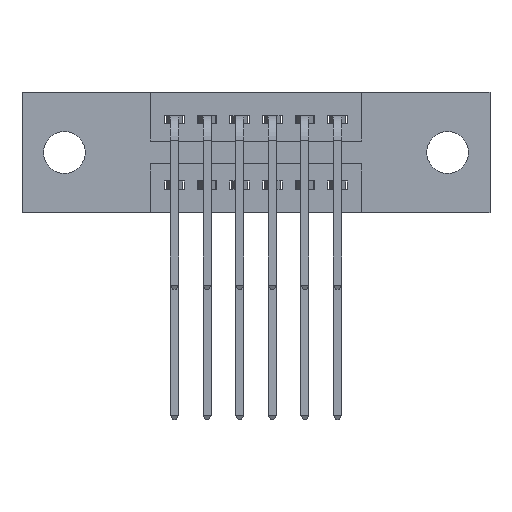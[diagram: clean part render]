
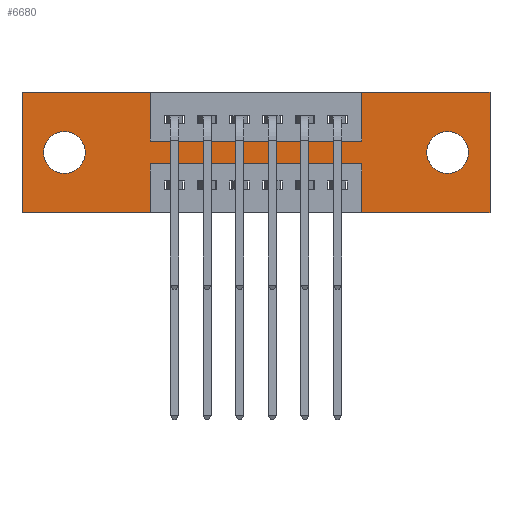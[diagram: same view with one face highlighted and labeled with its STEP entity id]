
A CAD part, front view. The second image highlights one B-rep face of the part: STEP entity #6680.
In plain terms, the highlighted planar face has unit normal (0, -1, 0).
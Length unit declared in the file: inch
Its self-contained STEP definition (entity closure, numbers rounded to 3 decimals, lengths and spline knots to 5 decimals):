
#110 = VERTEX_POINT ( 'NONE', #5980 ) ;
#482 = CARTESIAN_POINT ( 'NONE',  ( 0.13, 0., -0.249 ) ) ;
#796 = DIRECTION ( 'NONE',  ( 0., 0., 1. ) ) ;
#899 = EDGE_LOOP ( 'NONE', ( #6885, #7157 ) ) ;
#951 = DIRECTION ( 'NONE',  ( 0., 1., 0. ) ) ;
#990 = ORIENTED_EDGE ( 'NONE', *, *, #6257, .F. ) ;
#1080 = CARTESIAN_POINT ( 'NONE',  ( 1.305, 0., -0.185 ) ) ;
#1132 = VERTEX_POINT ( 'NONE', #8359 ) ;
#1253 = DIRECTION ( 'NONE',  ( 0., 0., -1. ) ) ;
#1435 = EDGE_LOOP ( 'NONE', ( #5346, #6732 ) ) ;
#1572 = AXIS2_PLACEMENT_3D ( 'NONE', #5475, #6610, #10519 ) ;
#1613 = VERTEX_POINT ( 'NONE', #11039 ) ;
#1637 = CARTESIAN_POINT ( 'NONE',  ( 0.3925, 0., -0.37 ) ) ;
#1645 = LINE ( 'NONE', #7746, #5873 ) ;
#1800 = VECTOR ( 'NONE', #2091, 39.37008 ) ;
#1890 = DIRECTION ( 'NONE',  ( 0., 0., 1. ) ) ;
#1992 = VECTOR ( 'NONE', #7218, 39.37008 ) ;
#2032 = VECTOR ( 'NONE', #8519, 39.37008 ) ;
#2034 = ORIENTED_EDGE ( 'NONE', *, *, #11187, .F. ) ;
#2044 = EDGE_CURVE ( 'NONE', #8488, #10544, #10368, .T. ) ;
#2058 = DIRECTION ( 'NONE',  ( 0., 0., -1. ) ) ;
#2091 = DIRECTION ( 'NONE',  ( 1., 0., 0. ) ) ;
#2223 = CARTESIAN_POINT ( 'NONE',  ( 1.435, 0., 0. ) ) ;
#2295 = VECTOR ( 'NONE', #4329, 39.37008 ) ;
#2473 = DIRECTION ( 'NONE',  ( 0., 0., -1. ) ) ;
#2516 = CARTESIAN_POINT ( 'NONE',  ( 0.13, 0., -0.121 ) ) ;
#2913 = PLANE ( 'NONE',  #1572 ) ;
#2925 = FACE_OUTER_BOUND ( 'NONE', #10430, .T. ) ;
#2967 = CIRCLE ( 'NONE', #6781, 0.064 ) ;
#2994 = VERTEX_POINT ( 'NONE', #9888 ) ;
#3142 = DIRECTION ( 'NONE',  ( 0., 0., 1. ) ) ;
#3173 = VECTOR ( 'NONE', #1890, 39.37008 ) ;
#3327 = CARTESIAN_POINT ( 'NONE',  ( 1.305, 0., -0.185 ) ) ;
#3368 = DIRECTION ( 'NONE',  ( 0., 1., 0. ) ) ;
#3375 = LINE ( 'NONE', #4186, #7590 ) ;
#3460 = LINE ( 'NONE', #7805, #3173 ) ;
#3472 = CARTESIAN_POINT ( 'NONE',  ( 0., 0., -0.37 ) ) ;
#3793 = ORIENTED_EDGE ( 'NONE', *, *, #10353, .F. ) ;
#3949 = AXIS2_PLACEMENT_3D ( 'NONE', #3327, #3368, #2473 ) ;
#4036 = VECTOR ( 'NONE', #6862, 39.37008 ) ;
#4050 = CARTESIAN_POINT ( 'NONE',  ( 0.13, 0., -0.185 ) ) ;
#4064 = CARTESIAN_POINT ( 'NONE',  ( 1.0425, 0., -0.37 ) ) ;
#4069 = ORIENTED_EDGE ( 'NONE', *, *, #7620, .F. ) ;
#4095 = LINE ( 'NONE', #4652, #1800 ) ;
#4186 = CARTESIAN_POINT ( 'NONE',  ( 0.3925, 0., -0.37 ) ) ;
#4329 = DIRECTION ( 'NONE',  ( -1., 0., 0. ) ) ;
#4341 = CARTESIAN_POINT ( 'NONE',  ( 0.3925, 0., -0.22 ) ) ;
#4430 = ORIENTED_EDGE ( 'NONE', *, *, #9631, .F. ) ;
#4598 = EDGE_CURVE ( 'NONE', #8013, #10363, #8521, .T. ) ;
#4652 = CARTESIAN_POINT ( 'NONE',  ( 0.3925, 0., -0.15 ) ) ;
#4670 = CIRCLE ( 'NONE', #8325, 0.064 ) ;
#4731 = CARTESIAN_POINT ( 'NONE',  ( 1.435, 0., 0. ) ) ;
#4863 = VECTOR ( 'NONE', #6016, 39.37008 ) ;
#4864 = DIRECTION ( 'NONE',  ( 0., 0., 1. ) ) ;
#4974 = VERTEX_POINT ( 'NONE', #9897 ) ;
#5029 = VERTEX_POINT ( 'NONE', #2516 ) ;
#5172 = ORIENTED_EDGE ( 'NONE', *, *, #10574, .F. ) ;
#5346 = ORIENTED_EDGE ( 'NONE', *, *, #10771, .T. ) ;
#5475 = CARTESIAN_POINT ( 'NONE',  ( 0., 0., -0.37 ) ) ;
#5684 = ORIENTED_EDGE ( 'NONE', *, *, #7367, .F. ) ;
#5700 = VECTOR ( 'NONE', #3142, 39.37008 ) ;
#5838 = DIRECTION ( 'NONE',  ( 0., 0., -1. ) ) ;
#5873 = VECTOR ( 'NONE', #796, 39.37008 ) ;
#5918 = CARTESIAN_POINT ( 'NONE',  ( 0.3925, 0., -0.22 ) ) ;
#5980 = CARTESIAN_POINT ( 'NONE',  ( 1.435, 0., -0.37 ) ) ;
#6016 = DIRECTION ( 'NONE',  ( 0., 0., -1. ) ) ;
#6097 = CARTESIAN_POINT ( 'NONE',  ( 0.13, 0., -0.185 ) ) ;
#6151 = VERTEX_POINT ( 'NONE', #4341 ) ;
#6163 = LINE ( 'NONE', #6328, #1992 ) ;
#6257 = EDGE_CURVE ( 'NONE', #1613, #7029, #6163, .T. ) ;
#6328 = CARTESIAN_POINT ( 'NONE',  ( 0., 0., 0. ) ) ;
#6338 = CIRCLE ( 'NONE', #10273, 0.064 ) ;
#6579 = CARTESIAN_POINT ( 'NONE',  ( 1.305, 0., -0.249 ) ) ;
#6610 = DIRECTION ( 'NONE',  ( 0., -1., 0. ) ) ;
#6680 = ADVANCED_FACE ( 'NONE', ( #7410, #9677, #2925 ), #2913, .T. ) ;
#6732 = ORIENTED_EDGE ( 'NONE', *, *, #2044, .T. ) ;
#6761 = ORIENTED_EDGE ( 'NONE', *, *, #10606, .F. ) ;
#6781 = AXIS2_PLACEMENT_3D ( 'NONE', #6097, #951, #6973 ) ;
#6862 = DIRECTION ( 'NONE',  ( 1., 0., 0. ) ) ;
#6885 = ORIENTED_EDGE ( 'NONE', *, *, #10942, .T. ) ;
#6973 = DIRECTION ( 'NONE',  ( 0., 0., 1. ) ) ;
#6996 = LINE ( 'NONE', #5918, #2295 ) ;
#7029 = VERTEX_POINT ( 'NONE', #2223 ) ;
#7072 = CARTESIAN_POINT ( 'NONE',  ( 0., 0., 0. ) ) ;
#7079 = DIRECTION ( 'NONE',  ( 0., 1., 0. ) ) ;
#7157 = ORIENTED_EDGE ( 'NONE', *, *, #10693, .T. ) ;
#7218 = DIRECTION ( 'NONE',  ( 1., 0., 0. ) ) ;
#7257 = CARTESIAN_POINT ( 'NONE',  ( 0.3925, 0., 0. ) ) ;
#7367 = EDGE_CURVE ( 'NONE', #8425, #4974, #1645, .T. ) ;
#7410 = FACE_BOUND ( 'NONE', #1435, .T. ) ;
#7451 = EDGE_CURVE ( 'NONE', #1132, #1613, #3460, .T. ) ;
#7590 = VECTOR ( 'NONE', #5838, 39.37008 ) ;
#7620 = EDGE_CURVE ( 'NONE', #2994, #1132, #4095, .T. ) ;
#7746 = CARTESIAN_POINT ( 'NONE',  ( 1.0425, 0., -0.37 ) ) ;
#7767 = LINE ( 'NONE', #8194, #5700 ) ;
#7805 = CARTESIAN_POINT ( 'NONE',  ( 1.0425, 0., 0. ) ) ;
#8013 = VERTEX_POINT ( 'NONE', #8542 ) ;
#8054 = EDGE_CURVE ( 'NONE', #10363, #2994, #9091, .T. ) ;
#8194 = CARTESIAN_POINT ( 'NONE',  ( 0., 0., 0. ) ) ;
#8256 = VECTOR ( 'NONE', #10271, 39.37008 ) ;
#8325 = AXIS2_PLACEMENT_3D ( 'NONE', #4050, #9963, #4864 ) ;
#8359 = CARTESIAN_POINT ( 'NONE',  ( 1.0425, 0., -0.15 ) ) ;
#8395 = VECTOR ( 'NONE', #1253, 39.37008 ) ;
#8425 = VERTEX_POINT ( 'NONE', #4064 ) ;
#8488 = VERTEX_POINT ( 'NONE', #6579 ) ;
#8519 = DIRECTION ( 'NONE',  ( -1., 0., 0. ) ) ;
#8521 = LINE ( 'NONE', #7072, #4036 ) ;
#8542 = CARTESIAN_POINT ( 'NONE',  ( 0., 0., 0. ) ) ;
#8552 = CARTESIAN_POINT ( 'NONE',  ( 0., 0., -0.37 ) ) ;
#8808 = ORIENTED_EDGE ( 'NONE', *, *, #4598, .F. ) ;
#9037 = LINE ( 'NONE', #3472, #2032 ) ;
#9057 = VERTEX_POINT ( 'NONE', #482 ) ;
#9091 = LINE ( 'NONE', #11194, #4863 ) ;
#9208 = ORIENTED_EDGE ( 'NONE', *, *, #7451, .F. ) ;
#9336 = CARTESIAN_POINT ( 'NONE',  ( 1.305, 0., -0.121 ) ) ;
#9631 = EDGE_CURVE ( 'NONE', #10315, #8013, #7767, .T. ) ;
#9677 = FACE_BOUND ( 'NONE', #899, .T. ) ;
#9774 = CARTESIAN_POINT ( 'NONE',  ( 0., 0., -0.37 ) ) ;
#9888 = CARTESIAN_POINT ( 'NONE',  ( 0.3925, 0., -0.15 ) ) ;
#9897 = CARTESIAN_POINT ( 'NONE',  ( 1.0425, 0., -0.22 ) ) ;
#9963 = DIRECTION ( 'NONE',  ( 0., 1., 0. ) ) ;
#10271 = DIRECTION ( 'NONE',  ( -1., 0., 0. ) ) ;
#10273 = AXIS2_PLACEMENT_3D ( 'NONE', #1080, #7079, #2058 ) ;
#10315 = VERTEX_POINT ( 'NONE', #9774 ) ;
#10353 = EDGE_CURVE ( 'NONE', #7029, #110, #10651, .T. ) ;
#10363 = VERTEX_POINT ( 'NONE', #7257 ) ;
#10368 = CIRCLE ( 'NONE', #3949, 0.064 ) ;
#10430 = EDGE_LOOP ( 'NONE', ( #10516, #2034, #5684, #5172, #3793, #990, #9208, #4069, #10533, #8808, #4430, #6761 ) ) ;
#10514 = LINE ( 'NONE', #8552, #8256 ) ;
#10516 = ORIENTED_EDGE ( 'NONE', *, *, #11055, .F. ) ;
#10519 = DIRECTION ( 'NONE',  ( 0., 0., -1. ) ) ;
#10533 = ORIENTED_EDGE ( 'NONE', *, *, #8054, .F. ) ;
#10542 = VERTEX_POINT ( 'NONE', #1637 ) ;
#10544 = VERTEX_POINT ( 'NONE', #9336 ) ;
#10574 = EDGE_CURVE ( 'NONE', #110, #8425, #9037, .T. ) ;
#10606 = EDGE_CURVE ( 'NONE', #10542, #10315, #10514, .T. ) ;
#10651 = LINE ( 'NONE', #4731, #8395 ) ;
#10693 = EDGE_CURVE ( 'NONE', #9057, #5029, #2967, .T. ) ;
#10771 = EDGE_CURVE ( 'NONE', #10544, #8488, #6338, .T. ) ;
#10942 = EDGE_CURVE ( 'NONE', #5029, #9057, #4670, .T. ) ;
#11039 = CARTESIAN_POINT ( 'NONE',  ( 1.0425, 0., 0. ) ) ;
#11055 = EDGE_CURVE ( 'NONE', #6151, #10542, #3375, .T. ) ;
#11187 = EDGE_CURVE ( 'NONE', #4974, #6151, #6996, .T. ) ;
#11194 = CARTESIAN_POINT ( 'NONE',  ( 0.3925, 0., 0. ) ) ;
